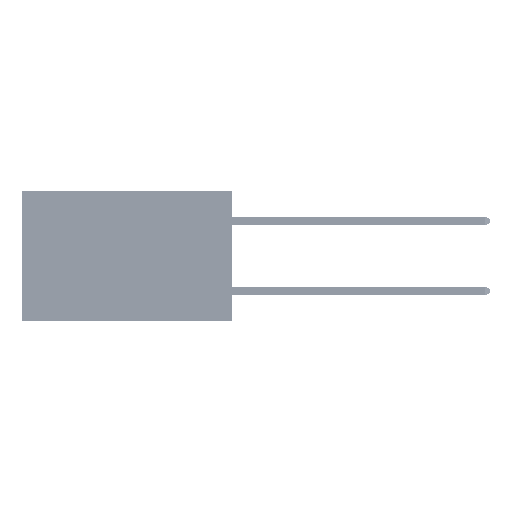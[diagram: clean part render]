
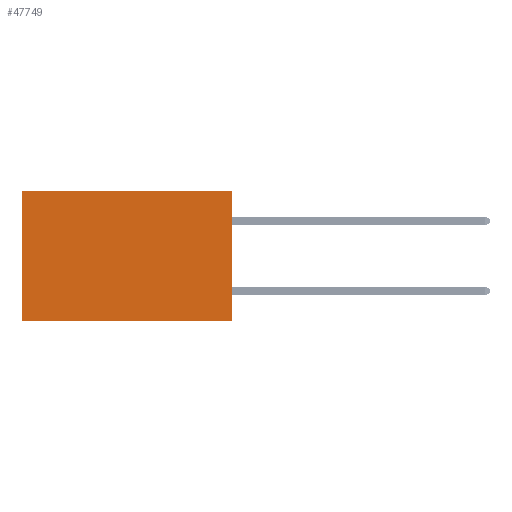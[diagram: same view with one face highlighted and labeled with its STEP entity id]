
A CAD part, left-side view. The second image highlights one B-rep face of the part: STEP entity #47749.
In plain terms, the highlighted planar face has unit normal (-1, 0, 0).
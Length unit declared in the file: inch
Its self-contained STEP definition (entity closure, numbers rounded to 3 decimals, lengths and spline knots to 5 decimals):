
#757 = PLANE ( 'NONE',  #43249 ) ;
#2850 = EDGE_CURVE ( 'NONE', #19020, #38219, #7256, .T. ) ;
#3034 = CARTESIAN_POINT ( 'NONE',  ( 0.2875, 0., 0. ) ) ;
#7256 = LINE ( 'NONE', #40818, #41412 ) ;
#7815 = VERTEX_POINT ( 'NONE', #10568 ) ;
#7983 = DIRECTION ( 'NONE',  ( 1., 0., 0. ) ) ;
#8167 = ORIENTED_EDGE ( 'NONE', *, *, #43359, .T. ) ;
#10568 = CARTESIAN_POINT ( 'NONE',  ( 0.2875, 0., 0. ) ) ;
#10893 = DIRECTION ( 'NONE',  ( 0., 0., -1. ) ) ;
#11468 = CARTESIAN_POINT ( 'NONE',  ( 0.2875, 0., 0. ) ) ;
#12097 = LINE ( 'NONE', #23586, #19738 ) ;
#13245 = EDGE_CURVE ( 'NONE', #28181, #38219, #33372, .T. ) ;
#13903 = CARTESIAN_POINT ( 'NONE',  ( 0.2875, 0., -0.37 ) ) ;
#14412 = VECTOR ( 'NONE', #10893, 39.37008 ) ;
#15244 = ORIENTED_EDGE ( 'NONE', *, *, #19100, .F. ) ;
#18117 = CARTESIAN_POINT ( 'NONE',  ( 0.2875, 0.6, -0.37 ) ) ;
#18434 = EDGE_LOOP ( 'NONE', ( #32906, #18662, #15244, #8167 ) ) ;
#18662 = ORIENTED_EDGE ( 'NONE', *, *, #2850, .F. ) ;
#18781 = CARTESIAN_POINT ( 'NONE',  ( 0.2875, 0.6, 0. ) ) ;
#19020 = VERTEX_POINT ( 'NONE', #13903 ) ;
#19100 = EDGE_CURVE ( 'NONE', #7815, #19020, #26143, .T. ) ;
#19738 = VECTOR ( 'NONE', #42038, 39.37008 ) ;
#23586 = CARTESIAN_POINT ( 'NONE',  ( 0.2875, 0., 0. ) ) ;
#25060 = DIRECTION ( 'NONE',  ( 0., 0., -1. ) ) ;
#25349 = CARTESIAN_POINT ( 'NONE',  ( 0.2875, 0.6, 0. ) ) ;
#26143 = LINE ( 'NONE', #3034, #14412 ) ;
#28181 = VERTEX_POINT ( 'NONE', #25349 ) ;
#29481 = FACE_OUTER_BOUND ( 'NONE', #18434, .T. ) ;
#32906 = ORIENTED_EDGE ( 'NONE', *, *, #13245, .T. ) ;
#33372 = LINE ( 'NONE', #18781, #34549 ) ;
#34549 = VECTOR ( 'NONE', #25060, 39.37008 ) ;
#38219 = VERTEX_POINT ( 'NONE', #18117 ) ;
#40818 = CARTESIAN_POINT ( 'NONE',  ( 0.2875, 0., -0.37 ) ) ;
#41412 = VECTOR ( 'NONE', #48555, 39.37008 ) ;
#41581 = DIRECTION ( 'NONE',  ( 0., 0., -1. ) ) ;
#42038 = DIRECTION ( 'NONE',  ( 0., 1., 0. ) ) ;
#43249 = AXIS2_PLACEMENT_3D ( 'NONE', #11468, #7983, #41581 ) ;
#43359 = EDGE_CURVE ( 'NONE', #7815, #28181, #12097, .T. ) ;
#47749 = ADVANCED_FACE ( 'NONE', ( #29481 ), #757, .F. ) ;
#48555 = DIRECTION ( 'NONE',  ( 0., 1., 0. ) ) ;
